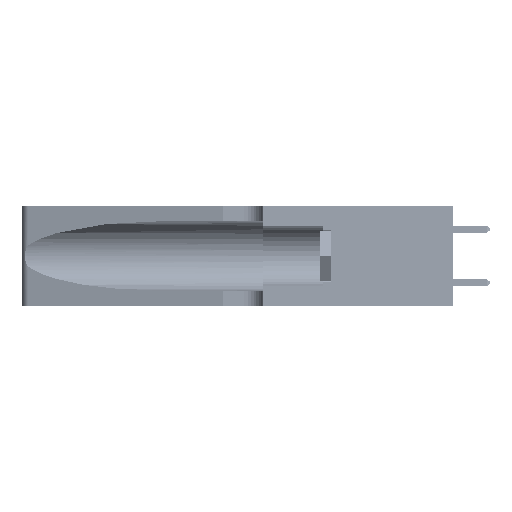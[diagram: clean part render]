
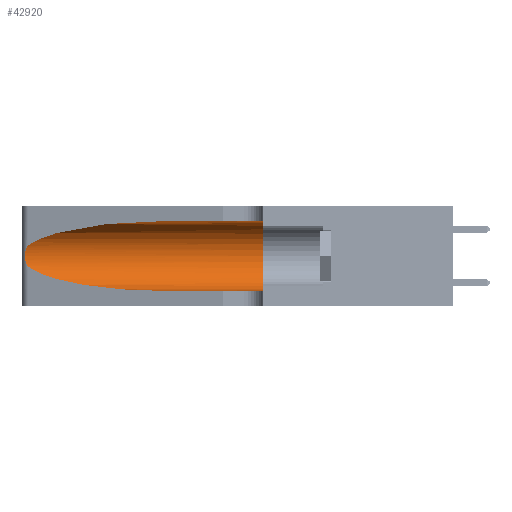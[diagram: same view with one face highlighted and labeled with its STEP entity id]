
A CAD part, left-side view. The second image highlights one B-rep face of the part: STEP entity #42920.
In plain terms, the highlighted cylindrical face has radius 3.308 mm (diameter 6.617 mm), a partial arc.
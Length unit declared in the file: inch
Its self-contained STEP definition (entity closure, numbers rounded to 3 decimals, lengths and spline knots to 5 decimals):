
#348 = CARTESIAN_POINT ( 'NONE',  ( 0.26075, 1.23896, 0.19203 ) ) ;
#572 = EDGE_CURVE ( 'NONE', #2603, #4949, #39320, .T. ) ;
#1489 = CARTESIAN_POINT ( 'NONE',  ( 0.1305, 0.35, 0.185 ) ) ;
#1987 = CARTESIAN_POINT ( 'NONE',  ( 0.1305, 1.61858, 0.31525 ) ) ;
#2118 = CIRCLE ( 'NONE', #36100, 0.13025 ) ;
#2603 = VERTEX_POINT ( 'NONE', #25878 ) ;
#2930 = ORIENTED_EDGE ( 'NONE', *, *, #31688, .F. ) ;
#4448 = CARTESIAN_POINT ( 'NONE',  ( 0.26017, 1.23833, 0.17102 ) ) ;
#4949 = VERTEX_POINT ( 'NONE', #24424 ) ;
#5602 = DIRECTION ( 'NONE',  ( 0., 0., 1. ) ) ;
#5961 = CARTESIAN_POINT ( 'NONE',  ( 0.2373, 1.15595, 0.28018 ) ) ;
#6795 = ORIENTED_EDGE ( 'NONE', *, *, #41616, .T. ) ;
#8568 = CARTESIAN_POINT ( 'NONE',  ( 0.25789, 1.23486, 0.15765 ) ) ;
#9677 = DIRECTION ( 'NONE',  ( 0., -1., 0. ) ) ;
#10068 = CARTESIAN_POINT ( 'NONE',  ( 0.1305, 0.72297, 0.31525 ) ) ;
#10874 = CARTESIAN_POINT ( 'NONE',  ( 0.18966, 0.96281, 0.05475 ) ) ;
#12683 = CARTESIAN_POINT ( 'NONE',  ( 0.25555, 1.22993, 0.14849 ) ) ;
#13540 = LINE ( 'NONE', #1987, #33985 ) ;
#16717 = CARTESIAN_POINT ( 'NONE',  ( 0.1305, 0.72297, 0.31525 ) ) ;
#18081 = CARTESIAN_POINT ( 'NONE',  ( 0.18966, 0.96281, 0.31525 ) ) ;
#19542 = B_SPLINE_CURVE_WITH_KNOTS ( 'NONE', 3,
 ( #36938, #49081, #45140, #20733, #49254, #24831, #348, #28933, #4448, #33014, #8568, #37125, #12683, #41207 ),
 .UNSPECIFIED., .F., .F.,
 ( 4, 2, 2, 2, 2, 2, 4 ),
 ( 0., 0.00027, 0.00053, 0.00107, 0.0016, 0.00187, 0.00214 ),
 .UNSPECIFIED. ) ;
#20299 = DIRECTION ( 'NONE',  ( 0., -1., 0. ) ) ;
#20733 = CARTESIAN_POINT ( 'NONE',  ( 0.25787, 1.23484, 0.2124 ) ) ;
#21574 = FACE_OUTER_BOUND ( 'NONE', #49773, .T. ) ;
#23350 = CARTESIAN_POINT ( 'NONE',  ( 0.1305, 0.35, 0.31525 ) ) ;
#24424 = CARTESIAN_POINT ( 'NONE',  ( 0.1305, 0.35, 0.05475 ) ) ;
#24831 = CARTESIAN_POINT ( 'NONE',  ( 0.26018, 1.23835, 0.19895 ) ) ;
#25267 = ORIENTED_EDGE ( 'NONE', *, *, #572, .T. ) ;
#25878 = CARTESIAN_POINT ( 'NONE',  ( 0.1305, 0.72297, 0.05475 ) ) ;
#25921 = CARTESIAN_POINT ( 'NONE',  ( 0.1305, 1.61858, 0.05475 ) ) ;
#25944 = AXIS2_PLACEMENT_3D ( 'NONE', #32422, #20299, #48828 ) ;
#25971 = VERTEX_POINT ( 'NONE', #23350 ) ;
#27233 = VECTOR ( 'NONE', #9677, 39.37008 ) ;
#28433 = EDGE_CURVE ( 'NONE', #44991, #42775, #35100, .T. ) ;
#28933 = CARTESIAN_POINT ( 'NONE',  ( 0.26075, 1.23896, 0.178 ) ) ;
#30078 = DIRECTION ( 'NONE',  ( 0., 1., 0. ) ) ;
#31199 = CARTESIAN_POINT ( 'NONE',  ( 0.2373, 1.15595, 0.08982 ) ) ;
#31688 = EDGE_CURVE ( 'NONE', #44991, #25971, #13540, .T. ) ;
#32422 = CARTESIAN_POINT ( 'NONE',  ( 0.1305, 1.61858, 0.185 ) ) ;
#33014 = CARTESIAN_POINT ( 'NONE',  ( 0.25856, 1.23593, 0.16098 ) ) ;
#33985 = VECTOR ( 'NONE', #34675, 39.37008 ) ;
#34675 = DIRECTION ( 'NONE',  ( 0., -1., 0. ) ) ;
#35100 =( BOUNDED_CURVE ( )  B_SPLINE_CURVE ( 3, ( #10068, #18081, #5961, #38595 ),
 .UNSPECIFIED., .F., .F. ) 
 B_SPLINE_CURVE_WITH_KNOTS ( ( 4, 4 ),
 ( 1.5708, 2.84003 ),
 .UNSPECIFIED. ) 
 CURVE ( )  GEOMETRIC_REPRESENTATION_ITEM ( )  RATIONAL_B_SPLINE_CURVE ( ( 1., 0.87, 0.87, 1. ) ) 
 REPRESENTATION_ITEM ( '' )  );
#35403 = ORIENTED_EDGE ( 'NONE', *, *, #49454, .T. ) ;
#35844 = CARTESIAN_POINT ( 'NONE',  ( 0.25487, 1.22718, 0.22369 ) ) ;
#36100 = AXIS2_PLACEMENT_3D ( 'NONE', #1489, #30078, #5602 ) ;
#36266 = ORIENTED_EDGE ( 'NONE', *, *, #28433, .T. ) ;
#36938 = CARTESIAN_POINT ( 'NONE',  ( 0.25487, 1.22718, 0.22369 ) ) ;
#37125 = CARTESIAN_POINT ( 'NONE',  ( 0.25639, 1.23186, 0.15144 ) ) ;
#38557 = VERTEX_POINT ( 'NONE', #44605 ) ;
#38595 = CARTESIAN_POINT ( 'NONE',  ( 0.25487, 1.22718, 0.22369 ) ) ;
#39320 = LINE ( 'NONE', #25921, #27233 ) ;
#39364 = CARTESIAN_POINT ( 'NONE',  ( 0.1305, 0.72297, 0.05475 ) ) ;
#39549 = EDGE_CURVE ( 'NONE', #25971, #4949, #2118, .T. ) ;
#41207 = CARTESIAN_POINT ( 'NONE',  ( 0.25487, 1.22718, 0.14631 ) ) ;
#41616 = EDGE_CURVE ( 'NONE', #42775, #38557, #19542, .T. ) ;
#42775 = VERTEX_POINT ( 'NONE', #35844 ) ;
#42920 = ADVANCED_FACE ( 'NONE', ( #21574 ), #51533, .F. ) ;
#44605 = CARTESIAN_POINT ( 'NONE',  ( 0.25487, 1.22718, 0.14631 ) ) ;
#44991 = VERTEX_POINT ( 'NONE', #16717 ) ;
#45140 = CARTESIAN_POINT ( 'NONE',  ( 0.25639, 1.23184, 0.21858 ) ) ;
#48492 =( BOUNDED_CURVE ( )  B_SPLINE_CURVE ( 3, ( #51518, #31199, #10874, #39364 ),
 .UNSPECIFIED., .F., .F. ) 
 B_SPLINE_CURVE_WITH_KNOTS ( ( 4, 4 ),
 ( 3.44316, 4.71239 ),
 .UNSPECIFIED. ) 
 CURVE ( )  GEOMETRIC_REPRESENTATION_ITEM ( )  RATIONAL_B_SPLINE_CURVE ( ( 1., 0.87, 0.87, 1. ) ) 
 REPRESENTATION_ITEM ( '' )  );
#48828 = DIRECTION ( 'NONE',  ( 0., 0., -1. ) ) ;
#49081 = CARTESIAN_POINT ( 'NONE',  ( 0.25555, 1.22994, 0.2215 ) ) ;
#49254 = CARTESIAN_POINT ( 'NONE',  ( 0.25854, 1.2359, 0.20912 ) ) ;
#49454 = EDGE_CURVE ( 'NONE', #38557, #2603, #48492, .T. ) ;
#49773 = EDGE_LOOP ( 'NONE', ( #36266, #6795, #35403, #25267, #50523, #2930 ) ) ;
#50523 = ORIENTED_EDGE ( 'NONE', *, *, #39549, .F. ) ;
#51518 = CARTESIAN_POINT ( 'NONE',  ( 0.25487, 1.22718, 0.14631 ) ) ;
#51533 = CYLINDRICAL_SURFACE ( 'NONE', #25944, 0.13025 ) ;
